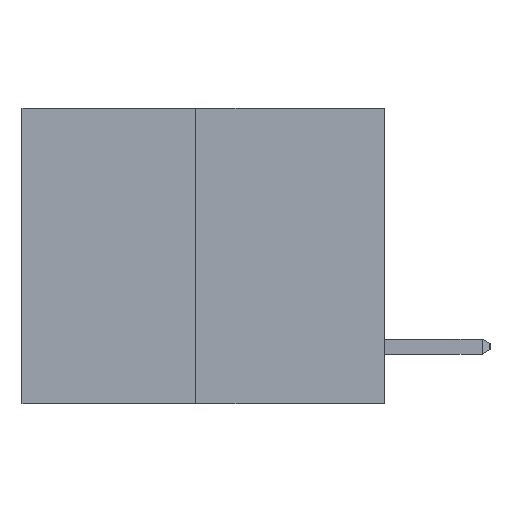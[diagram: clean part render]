
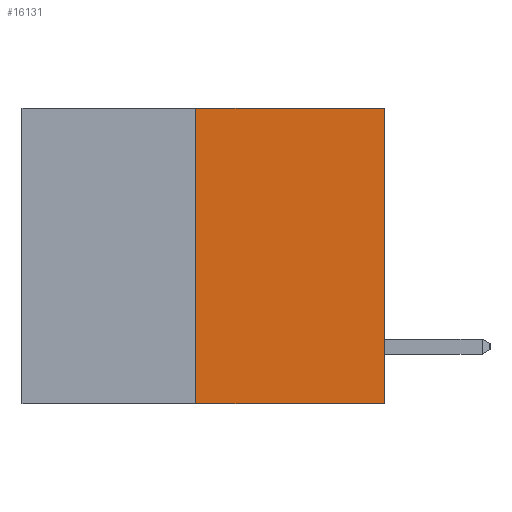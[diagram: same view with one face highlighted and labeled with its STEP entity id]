
A CAD part, left-side view. The second image highlights one B-rep face of the part: STEP entity #16131.
In plain terms, the highlighted planar face has unit normal (-1, 0, 0).
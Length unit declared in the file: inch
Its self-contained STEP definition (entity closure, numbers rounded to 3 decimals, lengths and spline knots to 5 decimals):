
#1738 = ORIENTED_EDGE ( 'NONE', *, *, #22868, .T. ) ;
#2290 = ORIENTED_EDGE ( 'NONE', *, *, #4244, .T. ) ;
#3124 = DIRECTION ( 'NONE',  ( 0., 0., -1. ) ) ;
#3802 = AXIS2_PLACEMENT_3D ( 'NONE', #18910, #13278, #3124 ) ;
#4244 = EDGE_CURVE ( 'NONE', #13283, #21065, #6357, .T. ) ;
#6136 = DIRECTION ( 'NONE',  ( 0., -1., 0. ) ) ;
#6357 = LINE ( 'NONE', #8626, #19430 ) ;
#7019 = DIRECTION ( 'NONE',  ( 0., 0., 1. ) ) ;
#7512 = VECTOR ( 'NONE', #10571, 39.37008 ) ;
#7684 = VECTOR ( 'NONE', #6136, 39.37008 ) ;
#8334 = CARTESIAN_POINT ( 'NONE',  ( 0., 0.312, -0.49 ) ) ;
#8626 = CARTESIAN_POINT ( 'NONE',  ( 0., 0., 0. ) ) ;
#9017 = VERTEX_POINT ( 'NONE', #14584 ) ;
#9246 = VECTOR ( 'NONE', #11762, 39.37008 ) ;
#9926 = ORIENTED_EDGE ( 'NONE', *, *, #15421, .F. ) ;
#10002 = LINE ( 'NONE', #10728, #7512 ) ;
#10531 = CARTESIAN_POINT ( 'NONE',  ( 0., 0., -0.49 ) ) ;
#10571 = DIRECTION ( 'NONE',  ( 0., 0., 1. ) ) ;
#10728 = CARTESIAN_POINT ( 'NONE',  ( 0., 0.312, -0.49 ) ) ;
#11762 = DIRECTION ( 'NONE',  ( 0., -1., 0. ) ) ;
#12518 = CARTESIAN_POINT ( 'NONE',  ( 0., 0., 0. ) ) ;
#12882 = ORIENTED_EDGE ( 'NONE', *, *, #19482, .F. ) ;
#13278 = DIRECTION ( 'NONE',  ( 1., 0., 0. ) ) ;
#13283 = VERTEX_POINT ( 'NONE', #10531 ) ;
#14584 = CARTESIAN_POINT ( 'NONE',  ( 0., 0.312, 0. ) ) ;
#15106 = LINE ( 'NONE', #15283, #9246 ) ;
#15283 = CARTESIAN_POINT ( 'NONE',  ( 0., 0.6, -0.49 ) ) ;
#15421 = EDGE_CURVE ( 'NONE', #18101, #9017, #10002, .T. ) ;
#16131 = ADVANCED_FACE ( 'NONE', ( #18879 ), #22160, .F. ) ;
#18101 = VERTEX_POINT ( 'NONE', #8334 ) ;
#18879 = FACE_OUTER_BOUND ( 'NONE', #22114, .T. ) ;
#18910 = CARTESIAN_POINT ( 'NONE',  ( 0., 0.6, 0. ) ) ;
#19430 = VECTOR ( 'NONE', #7019, 39.37008 ) ;
#19482 = EDGE_CURVE ( 'NONE', #9017, #21065, #22702, .T. ) ;
#21065 = VERTEX_POINT ( 'NONE', #12518 ) ;
#21656 = CARTESIAN_POINT ( 'NONE',  ( 0., 0.6, 0. ) ) ;
#22114 = EDGE_LOOP ( 'NONE', ( #9926, #1738, #2290, #12882 ) ) ;
#22160 = PLANE ( 'NONE',  #3802 ) ;
#22702 = LINE ( 'NONE', #21656, #7684 ) ;
#22868 = EDGE_CURVE ( 'NONE', #18101, #13283, #15106, .T. ) ;
